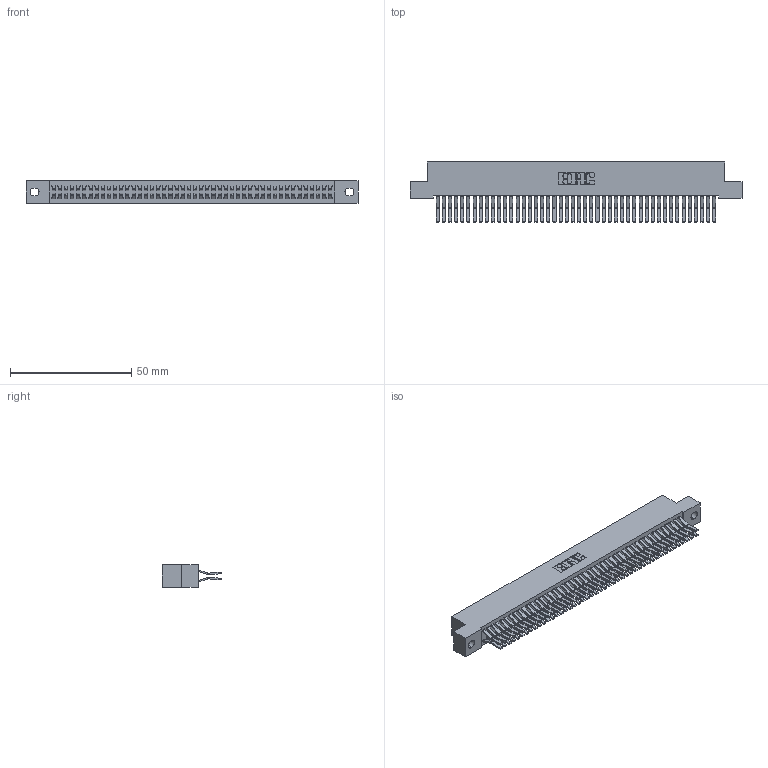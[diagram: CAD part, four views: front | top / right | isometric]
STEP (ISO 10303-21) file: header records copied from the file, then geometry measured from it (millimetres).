
FILE_DESCRIPTION (( 'STEP AP203' ), '1' );
FILE_NAME ('392-092-560-202.STEP', '2019-10-09T19:09:06', ( '' ), ( '' ), 'SwSTEP 2.0', 'SolidWorks 2016', '' );
FILE_SCHEMA (( 'CONFIG_CONTROL_DESIGN' ));
Length unit declared in the file: inch
Products named in the file (3): 342 Part_.128 Slot; 345-292-001_560 Tail; 392-092-560-202
Assembly tree (93 placements, depth 2):
  392-092-560-202
    342 Part_.128 Slot
    345-292-001_560 Tail  x92
Bounding box: 137.16 x 24.78 x 9.4 mm (x, y, z)
Volume: 12894.6 mm3; surface area: 22295.6 mm2
Topology: 93 solids, 93 shells, 5082 faces, 15123 edges, 9958 vertices
Faces by surface type: plane 3382, cylinder 1700
Entity records: 29167 total; most frequent: CARTESIAN_POINT 4830, ORIENTED_EDGE 4766, DIRECTION 4123, EDGE_CURVE 2383, VECTOR 2251, LINE 2251, VERTEX_POINT 1586, AXIS2_PLACEMENT_3D 936
